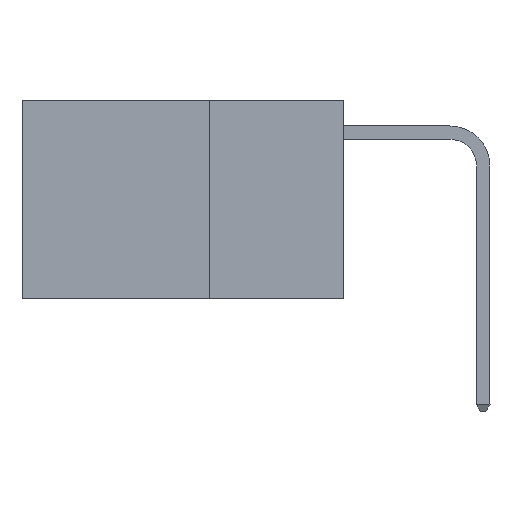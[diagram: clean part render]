
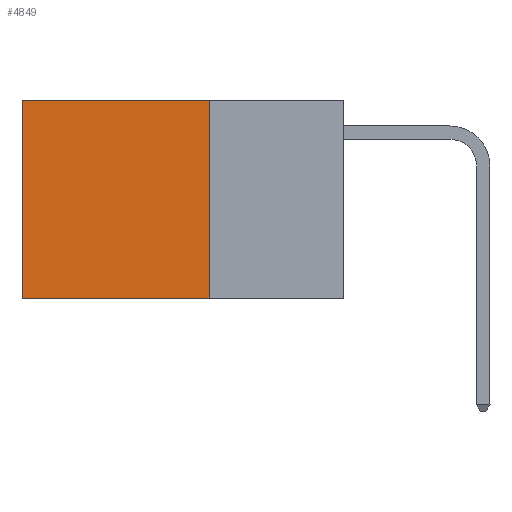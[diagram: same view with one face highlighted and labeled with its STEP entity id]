
A CAD part, left-side view. The second image highlights one B-rep face of the part: STEP entity #4849.
In plain terms, the highlighted planar face has unit normal (-1, 0, 0).
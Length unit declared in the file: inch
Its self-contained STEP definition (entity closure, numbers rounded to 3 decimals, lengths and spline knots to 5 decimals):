
#139 = ORIENTED_EDGE ( 'NONE', *, *, #2845, .T. ) ;
#230 = DIRECTION ( 'NONE',  ( 0., 0., -1. ) ) ;
#239 = DIRECTION ( 'NONE',  ( 0., 1., 0. ) ) ;
#269 = VERTEX_POINT ( 'NONE', #5295 ) ;
#288 = EDGE_CURVE ( 'NONE', #1767, #269, #4546, .T. ) ;
#662 = FACE_OUTER_BOUND ( 'NONE', #4555, .T. ) ;
#1123 = VECTOR ( 'NONE', #239, 39.37008 ) ;
#1126 = VECTOR ( 'NONE', #2701, 39.37008 ) ;
#1292 = DIRECTION ( 'NONE',  ( 0., 0., -1. ) ) ;
#1372 = PLANE ( 'NONE',  #8258 ) ;
#1767 = VERTEX_POINT ( 'NONE', #8188 ) ;
#1818 = VECTOR ( 'NONE', #7351, 39.37008 ) ;
#2116 = LINE ( 'NONE', #4860, #6449 ) ;
#2281 = ORIENTED_EDGE ( 'NONE', *, *, #8018, .F. ) ;
#2497 = ORIENTED_EDGE ( 'NONE', *, *, #288, .T. ) ;
#2701 = DIRECTION ( 'NONE',  ( 0., 0., -1. ) ) ;
#2845 = EDGE_CURVE ( 'NONE', #269, #4352, #2116, .T. ) ;
#2955 = LINE ( 'NONE', #5825, #1123 ) ;
#3423 = DIRECTION ( 'NONE',  ( 1., 0., 0. ) ) ;
#4005 = VERTEX_POINT ( 'NONE', #5627 ) ;
#4352 = VERTEX_POINT ( 'NONE', #7328 ) ;
#4546 = LINE ( 'NONE', #7402, #1818 ) ;
#4555 = EDGE_LOOP ( 'NONE', ( #139, #2281, #4911, #2497 ) ) ;
#4849 = ADVANCED_FACE ( 'NONE', ( #662 ), #1372, .F. ) ;
#4860 = CARTESIAN_POINT ( 'NONE',  ( 0.2625, 0.6, 0. ) ) ;
#4911 = ORIENTED_EDGE ( 'NONE', *, *, #8142, .F. ) ;
#5295 = CARTESIAN_POINT ( 'NONE',  ( 0.2625, 0.6, 0. ) ) ;
#5627 = CARTESIAN_POINT ( 'NONE',  ( 0.2625, 0.25, -0.37 ) ) ;
#5825 = CARTESIAN_POINT ( 'NONE',  ( 0.2625, 0.25, -0.37 ) ) ;
#6449 = VECTOR ( 'NONE', #230, 39.37008 ) ;
#6873 = LINE ( 'NONE', #9003, #1126 ) ;
#7328 = CARTESIAN_POINT ( 'NONE',  ( 0.2625, 0.6, -0.37 ) ) ;
#7351 = DIRECTION ( 'NONE',  ( 0., 1., 0. ) ) ;
#7402 = CARTESIAN_POINT ( 'NONE',  ( 0.2625, 0.25, 0. ) ) ;
#7585 = CARTESIAN_POINT ( 'NONE',  ( 0.2625, 0.25, 0. ) ) ;
#8018 = EDGE_CURVE ( 'NONE', #4005, #4352, #2955, .T. ) ;
#8142 = EDGE_CURVE ( 'NONE', #1767, #4005, #6873, .T. ) ;
#8188 = CARTESIAN_POINT ( 'NONE',  ( 0.2625, 0.25, 0. ) ) ;
#8258 = AXIS2_PLACEMENT_3D ( 'NONE', #7585, #3423, #1292 ) ;
#9003 = CARTESIAN_POINT ( 'NONE',  ( 0.2625, 0.25, 0. ) ) ;
